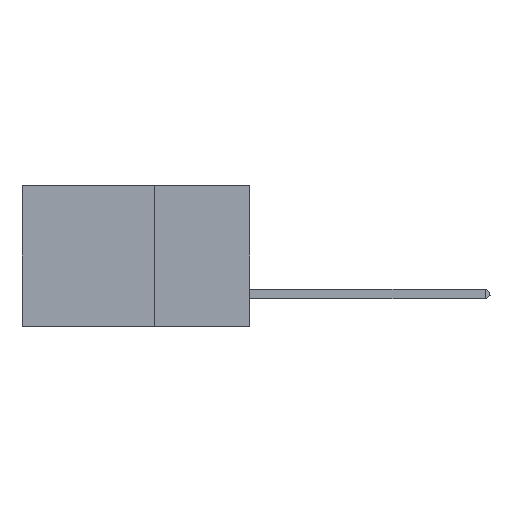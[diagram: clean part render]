
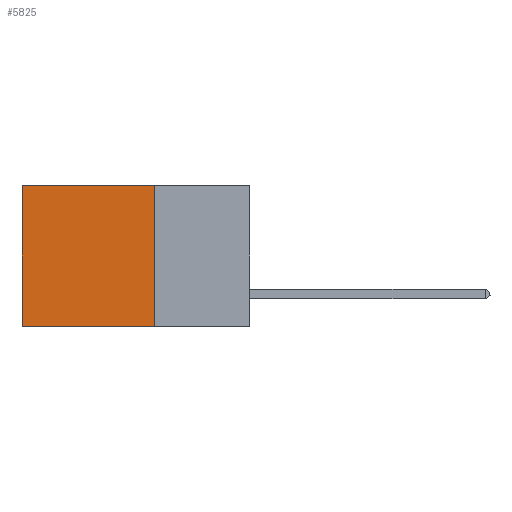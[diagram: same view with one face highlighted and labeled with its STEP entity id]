
A CAD part, left-side view. The second image highlights one B-rep face of the part: STEP entity #5825.
In plain terms, the highlighted planar face has unit normal (-1, 0, 0).
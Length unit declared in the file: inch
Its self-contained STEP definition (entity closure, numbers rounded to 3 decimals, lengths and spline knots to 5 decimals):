
#691 = VERTEX_POINT ( 'NONE', #18431 ) ;
#726 = DIRECTION ( 'NONE',  ( 1., 0., 0. ) ) ;
#761 = CARTESIAN_POINT ( 'NONE',  ( 0.2875, 0.25, -0.37 ) ) ;
#1463 = CARTESIAN_POINT ( 'NONE',  ( 0.2875, 0.6, 0. ) ) ;
#2650 = CARTESIAN_POINT ( 'NONE',  ( 0.2875, 0.25, -0.37 ) ) ;
#3150 = ORIENTED_EDGE ( 'NONE', *, *, #9285, .F. ) ;
#4010 = PLANE ( 'NONE',  #7295 ) ;
#4287 = VERTEX_POINT ( 'NONE', #2650 ) ;
#5825 = ADVANCED_FACE ( 'NONE', ( #6978 ), #4010, .F. ) ;
#5835 = LINE ( 'NONE', #1463, #15860 ) ;
#6396 = VECTOR ( 'NONE', #17574, 39.37008 ) ;
#6978 = FACE_OUTER_BOUND ( 'NONE', #14118, .T. ) ;
#7102 = VECTOR ( 'NONE', #16486, 39.37008 ) ;
#7195 = CARTESIAN_POINT ( 'NONE',  ( 0.2875, 0.25, 0. ) ) ;
#7295 = AXIS2_PLACEMENT_3D ( 'NONE', #7195, #726, #11988 ) ;
#7810 = ORIENTED_EDGE ( 'NONE', *, *, #20919, .T. ) ;
#9285 = EDGE_CURVE ( 'NONE', #4287, #691, #18091, .T. ) ;
#9937 = CARTESIAN_POINT ( 'NONE',  ( 0.2875, 0.25, 0. ) ) ;
#10878 = VECTOR ( 'NONE', #12096, 39.37008 ) ;
#11328 = VERTEX_POINT ( 'NONE', #19064 ) ;
#11723 = VERTEX_POINT ( 'NONE', #16176 ) ;
#11988 = DIRECTION ( 'NONE',  ( 0., 0., -1. ) ) ;
#12096 = DIRECTION ( 'NONE',  ( 0., 1., 0. ) ) ;
#12800 = DIRECTION ( 'NONE',  ( 0., 0., -1. ) ) ;
#12980 = LINE ( 'NONE', #9937, #7102 ) ;
#14039 = ORIENTED_EDGE ( 'NONE', *, *, #15619, .F. ) ;
#14118 = EDGE_LOOP ( 'NONE', ( #7810, #3150, #14039, #19398 ) ) ;
#15619 = EDGE_CURVE ( 'NONE', #11723, #4287, #17162, .T. ) ;
#15860 = VECTOR ( 'NONE', #12800, 39.37008 ) ;
#16143 = CARTESIAN_POINT ( 'NONE',  ( 0.2875, 0.25, 0. ) ) ;
#16176 = CARTESIAN_POINT ( 'NONE',  ( 0.2875, 0.25, 0. ) ) ;
#16486 = DIRECTION ( 'NONE',  ( 0., 1., 0. ) ) ;
#16696 = EDGE_CURVE ( 'NONE', #11723, #11328, #12980, .T. ) ;
#17162 = LINE ( 'NONE', #16143, #6396 ) ;
#17574 = DIRECTION ( 'NONE',  ( 0., 0., -1. ) ) ;
#18091 = LINE ( 'NONE', #761, #10878 ) ;
#18431 = CARTESIAN_POINT ( 'NONE',  ( 0.2875, 0.6, -0.37 ) ) ;
#19064 = CARTESIAN_POINT ( 'NONE',  ( 0.2875, 0.6, 0. ) ) ;
#19398 = ORIENTED_EDGE ( 'NONE', *, *, #16696, .T. ) ;
#20919 = EDGE_CURVE ( 'NONE', #11328, #691, #5835, .T. ) ;
